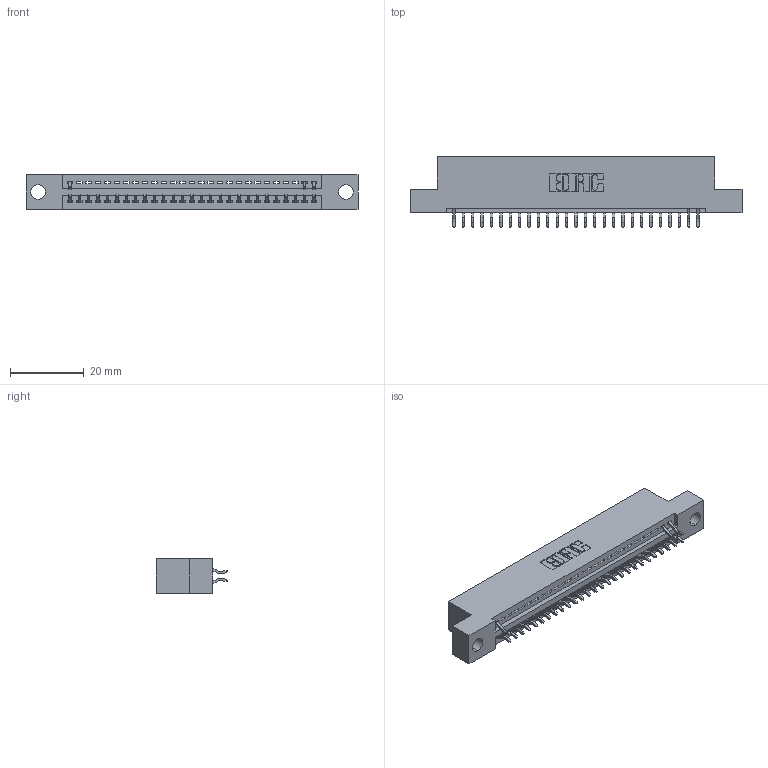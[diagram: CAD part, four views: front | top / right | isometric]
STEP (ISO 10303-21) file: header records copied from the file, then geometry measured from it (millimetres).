
FILE_DESCRIPTION (( 'STEP AP203' ), '1' );
FILE_NAME ('345-054-556-204.STEP', '2018-09-24T00:42:05', ( '' ), ( '' ), 'SwSTEP 2.0', 'SolidWorks 2016', '' );
FILE_SCHEMA (( 'CONFIG_CONTROL_DESIGN' ));
Length unit declared in the file: inch
Products named in the file (3): 345 Part_Flush Mounting Lugs - 0.156 Dia-TH; 345-292-001_556 Tail; 345-054-556-204
Assembly tree (31 placements, depth 2):
  345-054-556-204
    345 Part_Flush Mounting Lugs - 0.156 Dia-TH
    345-292-001_556 Tail  x30
Bounding box: 89.79 x 19.24 x 9.4 mm (x, y, z)
Volume: 8277.6 mm3; surface area: 10508.7 mm2
Topology: 31 solids, 31 shells, 1998 faces, 5999 edges, 3958 vertices
Faces by surface type: plane 1358, cylinder 640
Entity records: 22659 total; most frequent: CARTESIAN_POINT 3932, ORIENTED_EDGE 3878, DIRECTION 3447, EDGE_CURVE 1939, VECTOR 1691, LINE 1691, VERTEX_POINT 1290, AXIS2_PLACEMENT_3D 878
